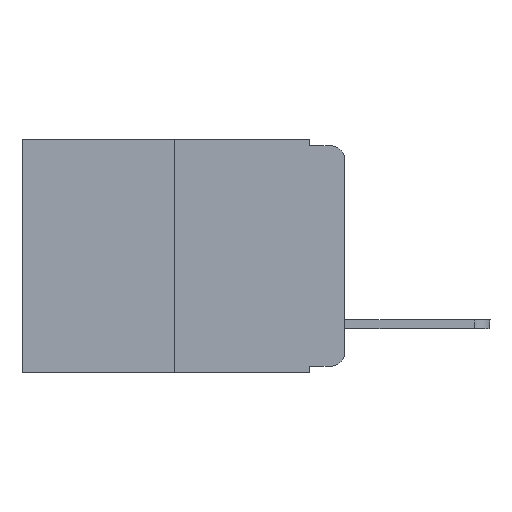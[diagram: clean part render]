
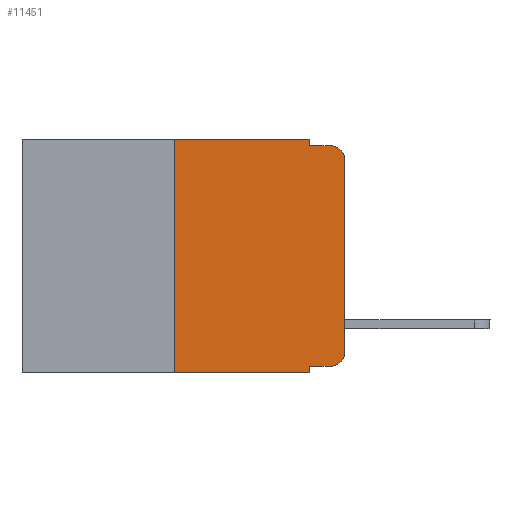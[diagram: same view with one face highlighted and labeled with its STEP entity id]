
A CAD part, left-side view. The second image highlights one B-rep face of the part: STEP entity #11451.
In plain terms, the highlighted planar face has unit normal (-1, 0, 0).
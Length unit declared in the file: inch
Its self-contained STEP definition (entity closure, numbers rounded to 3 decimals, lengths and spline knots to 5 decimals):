
#834 = CARTESIAN_POINT ( 'NONE',  ( 0., 0.25, -0.343 ) ) ;
#1092 = EDGE_CURVE ( 'NONE', #6023, #10670, #10728, .T. ) ;
#1269 = DIRECTION ( 'NONE',  ( 0., 0., -1. ) ) ;
#1285 = DIRECTION ( 'NONE',  ( 0., -1., 0. ) ) ;
#1709 = VECTOR ( 'NONE', #7179, 39.37008 ) ;
#1719 = VECTOR ( 'NONE', #17096, 39.37008 ) ;
#1852 = FACE_OUTER_BOUND ( 'NONE', #10366, .T. ) ;
#1940 = VERTEX_POINT ( 'NONE', #6006 ) ;
#2014 = VERTEX_POINT ( 'NONE', #13503 ) ;
#2444 = CARTESIAN_POINT ( 'NONE',  ( 0., 0., -0.03 ) ) ;
#2730 = DIRECTION ( 'NONE',  ( 0., 0., -1. ) ) ;
#2786 = LINE ( 'NONE', #17266, #11109 ) ;
#3391 = EDGE_CURVE ( 'NONE', #6692, #13670, #2786, .T. ) ;
#3508 = DIRECTION ( 'NONE',  ( 0., 0., -1. ) ) ;
#3766 = PLANE ( 'NONE',  #5097 ) ;
#4215 = CARTESIAN_POINT ( 'NONE',  ( 0., 0.02, -0.313 ) ) ;
#4287 = CARTESIAN_POINT ( 'NONE',  ( 0., 0.473, -0.343 ) ) ;
#4876 = EDGE_CURVE ( 'NONE', #1940, #2014, #14583, .T. ) ;
#5097 = AXIS2_PLACEMENT_3D ( 'NONE', #16790, #18206, #3508 ) ;
#5397 = VERTEX_POINT ( 'NONE', #2444 ) ;
#5404 = ORIENTED_EDGE ( 'NONE', *, *, #19095, .T. ) ;
#5506 = EDGE_CURVE ( 'NONE', #5397, #17643, #6278, .T. ) ;
#5675 = LINE ( 'NONE', #4287, #8252 ) ;
#6006 = CARTESIAN_POINT ( 'NONE',  ( 0., 0.02, -0.333 ) ) ;
#6023 = VERTEX_POINT ( 'NONE', #834 ) ;
#6047 = EDGE_CURVE ( 'NONE', #13670, #17643, #8584, .T. ) ;
#6278 = CIRCLE ( 'NONE', #9967, 0.02 ) ;
#6514 = VERTEX_POINT ( 'NONE', #9289 ) ;
#6587 = CARTESIAN_POINT ( 'NONE',  ( 0., 0.25, 0. ) ) ;
#6692 = VERTEX_POINT ( 'NONE', #15631 ) ;
#6790 = CARTESIAN_POINT ( 'NONE',  ( 0., 0.473, 0. ) ) ;
#6862 = VECTOR ( 'NONE', #13802, 39.37008 ) ;
#7179 = DIRECTION ( 'NONE',  ( 0., 0., 1. ) ) ;
#7363 = LINE ( 'NONE', #11565, #9428 ) ;
#7676 = CARTESIAN_POINT ( 'NONE',  ( 0., 0.051, -0.01 ) ) ;
#7755 = ORIENTED_EDGE ( 'NONE', *, *, #6047, .F. ) ;
#7959 = ORIENTED_EDGE ( 'NONE', *, *, #18016, .F. ) ;
#8252 = VECTOR ( 'NONE', #1285, 39.37008 ) ;
#8584 = LINE ( 'NONE', #18570, #17313 ) ;
#8673 = DIRECTION ( 'NONE',  ( -1., 0., 0. ) ) ;
#9289 = CARTESIAN_POINT ( 'NONE',  ( 0., 0.051, -0.333 ) ) ;
#9296 = EDGE_CURVE ( 'NONE', #10670, #6692, #9623, .T. ) ;
#9428 = VECTOR ( 'NONE', #2730, 39.37008 ) ;
#9461 = CARTESIAN_POINT ( 'NONE',  ( 0., 0.25, 0. ) ) ;
#9498 = DIRECTION ( 'NONE',  ( 0., -1., 0. ) ) ;
#9623 = LINE ( 'NONE', #6790, #1719 ) ;
#9756 = DIRECTION ( 'NONE',  ( 0., -1., 0. ) ) ;
#9967 = AXIS2_PLACEMENT_3D ( 'NONE', #12824, #8673, #1269 ) ;
#10366 = EDGE_LOOP ( 'NONE', ( #16006, #18711, #7755, #14313, #13775, #12413, #5404, #7959, #16063, #12670 ) ) ;
#10619 = CARTESIAN_POINT ( 'NONE',  ( 0., 0.02, -0.01 ) ) ;
#10664 = AXIS2_PLACEMENT_3D ( 'NONE', #4215, #13154, #17551 ) ;
#10670 = VERTEX_POINT ( 'NONE', #6587 ) ;
#10728 = LINE ( 'NONE', #9461, #6862 ) ;
#10736 = VECTOR ( 'NONE', #9498, 39.37008 ) ;
#10949 = CARTESIAN_POINT ( 'NONE',  ( 0., 0.051, -0.333 ) ) ;
#11109 = VECTOR ( 'NONE', #17205, 39.37008 ) ;
#11451 = ADVANCED_FACE ( 'NONE', ( #1852 ), #3766, .F. ) ;
#11565 = CARTESIAN_POINT ( 'NONE',  ( 0., 0.051, 0. ) ) ;
#11694 = CARTESIAN_POINT ( 'NONE',  ( 0., 0., 0. ) ) ;
#12342 = LINE ( 'NONE', #11694, #1709 ) ;
#12413 = ORIENTED_EDGE ( 'NONE', *, *, #1092, .F. ) ;
#12670 = ORIENTED_EDGE ( 'NONE', *, *, #4876, .T. ) ;
#12824 = CARTESIAN_POINT ( 'NONE',  ( 0., 0.02, -0.03 ) ) ;
#13154 = DIRECTION ( 'NONE',  ( -1., 0., 0. ) ) ;
#13503 = CARTESIAN_POINT ( 'NONE',  ( 0., 0., -0.313 ) ) ;
#13670 = VERTEX_POINT ( 'NONE', #7676 ) ;
#13775 = ORIENTED_EDGE ( 'NONE', *, *, #9296, .F. ) ;
#13802 = DIRECTION ( 'NONE',  ( 0., 0., 1. ) ) ;
#14262 = VERTEX_POINT ( 'NONE', #18035 ) ;
#14313 = ORIENTED_EDGE ( 'NONE', *, *, #3391, .F. ) ;
#14333 = EDGE_CURVE ( 'NONE', #6514, #1940, #15833, .T. ) ;
#14583 = CIRCLE ( 'NONE', #10664, 0.02 ) ;
#14645 = EDGE_CURVE ( 'NONE', #2014, #5397, #12342, .T. ) ;
#15631 = CARTESIAN_POINT ( 'NONE',  ( 0., 0.051, 0. ) ) ;
#15833 = LINE ( 'NONE', #10949, #10736 ) ;
#16006 = ORIENTED_EDGE ( 'NONE', *, *, #14645, .T. ) ;
#16063 = ORIENTED_EDGE ( 'NONE', *, *, #14333, .T. ) ;
#16790 = CARTESIAN_POINT ( 'NONE',  ( 0., 0.473, 0. ) ) ;
#17096 = DIRECTION ( 'NONE',  ( 0., -1., 0. ) ) ;
#17205 = DIRECTION ( 'NONE',  ( 0., 0., -1. ) ) ;
#17266 = CARTESIAN_POINT ( 'NONE',  ( 0., 0.051, 0. ) ) ;
#17313 = VECTOR ( 'NONE', #9756, 39.37008 ) ;
#17551 = DIRECTION ( 'NONE',  ( 0., 0., -1. ) ) ;
#17643 = VERTEX_POINT ( 'NONE', #10619 ) ;
#18016 = EDGE_CURVE ( 'NONE', #6514, #14262, #7363, .T. ) ;
#18035 = CARTESIAN_POINT ( 'NONE',  ( 0., 0.051, -0.343 ) ) ;
#18206 = DIRECTION ( 'NONE',  ( 1., 0., 0. ) ) ;
#18570 = CARTESIAN_POINT ( 'NONE',  ( 0., 0.051, -0.01 ) ) ;
#18711 = ORIENTED_EDGE ( 'NONE', *, *, #5506, .T. ) ;
#19095 = EDGE_CURVE ( 'NONE', #6023, #14262, #5675, .T. ) ;
